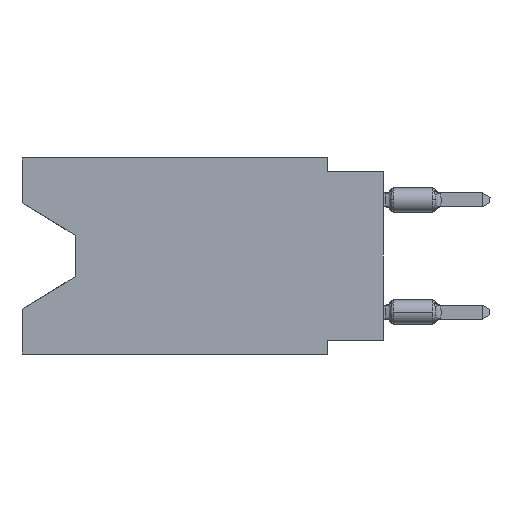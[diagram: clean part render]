
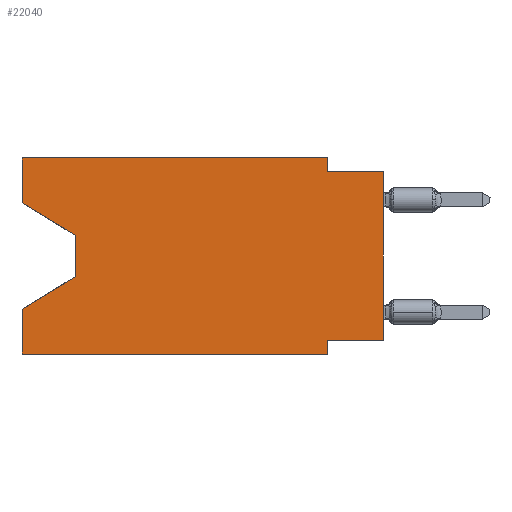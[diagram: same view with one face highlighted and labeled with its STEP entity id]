
A CAD part, left-side view. The second image highlights one B-rep face of the part: STEP entity #22040.
In plain terms, the highlighted planar face has unit normal (-1, 0, 0).
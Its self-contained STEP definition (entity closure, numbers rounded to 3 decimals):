
#743 = LINE ( 'NONE', #22579, #3223 ) ;
#1046 = LINE ( 'NONE', #13971, #13525 ) ;
#1055 = DIRECTION ( 'NONE',  ( 0., 0., 1. ) ) ;
#1995 = CARTESIAN_POINT ( 'NONE',  ( 0., 13.97, -5.385 ) ) ;
#2092 = CARTESIAN_POINT ( 'NONE',  ( 0., 16.383, 0. ) ) ;
#3223 = VECTOR ( 'NONE', #13660, 1000. ) ;
#3975 = LINE ( 'NONE', #13442, #32013 ) ;
#5871 = VERTEX_POINT ( 'NONE', #17220 ) ;
#7125 = ORIENTED_EDGE ( 'NONE', *, *, #10745, .T. ) ;
#7654 = VERTEX_POINT ( 'NONE', #24967 ) ;
#7940 = LINE ( 'NONE', #12248, #30791 ) ;
#9077 = LINE ( 'NONE', #12533, #16347 ) ;
#10044 = LINE ( 'NONE', #1995, #44112 ) ;
#10261 = ORIENTED_EDGE ( 'NONE', *, *, #47076, .T. ) ;
#10383 = CARTESIAN_POINT ( 'NONE',  ( 0., 16.383, -2.038 ) ) ;
#10745 = EDGE_CURVE ( 'NONE', #7654, #51484, #31964, .T. ) ;
#10991 = CARTESIAN_POINT ( 'NONE',  ( 0., 13.97, -3.505 ) ) ;
#11310 = CARTESIAN_POINT ( 'NONE',  ( 0., 2.54, 0. ) ) ;
#11563 = FACE_OUTER_BOUND ( 'NONE', #49711, .T. ) ;
#11608 = EDGE_CURVE ( 'NONE', #16523, #5871, #26941, .T. ) ;
#11979 = EDGE_CURVE ( 'NONE', #12028, #37269, #38691, .T. ) ;
#12028 = VERTEX_POINT ( 'NONE', #27717 ) ;
#12189 = CARTESIAN_POINT ( 'NONE',  ( 0., 2.54, -8.89 ) ) ;
#12248 = CARTESIAN_POINT ( 'NONE',  ( 0., 13.97, -3.505 ) ) ;
#12375 = EDGE_CURVE ( 'NONE', #30018, #5871, #10044, .T. ) ;
#12533 = CARTESIAN_POINT ( 'NONE',  ( 0., 16.383, 0. ) ) ;
#13442 = CARTESIAN_POINT ( 'NONE',  ( 0., 16.383, -8.89 ) ) ;
#13525 = VECTOR ( 'NONE', #22609, 1000. ) ;
#13660 = DIRECTION ( 'NONE',  ( 0., 0., 1. ) ) ;
#13665 = VECTOR ( 'NONE', #18730, 1000. ) ;
#13971 = CARTESIAN_POINT ( 'NONE',  ( 0., 0., -0.635 ) ) ;
#14748 = VERTEX_POINT ( 'NONE', #36480 ) ;
#15132 = EDGE_CURVE ( 'NONE', #36740, #51704, #41523, .T. ) ;
#15177 = EDGE_CURVE ( 'NONE', #12028, #49351, #51824, .T. ) ;
#15299 = DIRECTION ( 'NONE',  ( 1., 0., 0. ) ) ;
#16347 = VECTOR ( 'NONE', #16834, 1000. ) ;
#16513 = VECTOR ( 'NONE', #43290, 1000. ) ;
#16523 = VERTEX_POINT ( 'NONE', #43862 ) ;
#16834 = DIRECTION ( 'NONE',  ( 0., -1., 0. ) ) ;
#17220 = CARTESIAN_POINT ( 'NONE',  ( 0., 16.383, -6.852 ) ) ;
#18730 = DIRECTION ( 'NONE',  ( 0., -0.855, -0.519 ) ) ;
#19889 = ORIENTED_EDGE ( 'NONE', *, *, #15177, .T. ) ;
#20118 = VERTEX_POINT ( 'NONE', #34436 ) ;
#20897 = DIRECTION ( 'NONE',  ( 0., 0., -1. ) ) ;
#21114 = VECTOR ( 'NONE', #1055, 1000. ) ;
#22040 = ADVANCED_FACE ( 'NONE', ( #11563 ), #45507, .F. ) ;
#22579 = CARTESIAN_POINT ( 'NONE',  ( 0., 16.383, 0. ) ) ;
#22609 = DIRECTION ( 'NONE',  ( 0., -1., 0. ) ) ;
#24967 = CARTESIAN_POINT ( 'NONE',  ( 0., 16.383, -2.038 ) ) ;
#25403 = EDGE_CURVE ( 'NONE', #14748, #36740, #9077, .T. ) ;
#25697 = LINE ( 'NONE', #12189, #38447 ) ;
#26826 = VECTOR ( 'NONE', #52378, 1000. ) ;
#26941 = LINE ( 'NONE', #49068, #21114 ) ;
#27717 = CARTESIAN_POINT ( 'NONE',  ( 0., 0., -8.255 ) ) ;
#29427 = DIRECTION ( 'NONE',  ( 0., 0., -1. ) ) ;
#30018 = VERTEX_POINT ( 'NONE', #49094 ) ;
#30714 = EDGE_CURVE ( 'NONE', #37269, #20118, #25697, .T. ) ;
#30791 = VECTOR ( 'NONE', #20897, 1000. ) ;
#31431 = VECTOR ( 'NONE', #29427, 1000. ) ;
#31696 = ORIENTED_EDGE ( 'NONE', *, *, #25403, .F. ) ;
#31826 = AXIS2_PLACEMENT_3D ( 'NONE', #2092, #15299, #37749 ) ;
#31964 = LINE ( 'NONE', #10383, #13665 ) ;
#32013 = VECTOR ( 'NONE', #48527, 1000. ) ;
#34436 = CARTESIAN_POINT ( 'NONE',  ( 0., 2.54, -8.89 ) ) ;
#36480 = CARTESIAN_POINT ( 'NONE',  ( 0., 16.383, 0. ) ) ;
#36733 = ORIENTED_EDGE ( 'NONE', *, *, #11979, .F. ) ;
#36740 = VERTEX_POINT ( 'NONE', #53303 ) ;
#37269 = VERTEX_POINT ( 'NONE', #46584 ) ;
#37749 = DIRECTION ( 'NONE',  ( 0., 0., -1. ) ) ;
#38447 = VECTOR ( 'NONE', #42710, 1000. ) ;
#38691 = LINE ( 'NONE', #56780, #16513 ) ;
#38967 = EDGE_CURVE ( 'NONE', #7654, #14748, #743, .T. ) ;
#39242 = ORIENTED_EDGE ( 'NONE', *, *, #12375, .T. ) ;
#41523 = LINE ( 'NONE', #11310, #31431 ) ;
#42710 = DIRECTION ( 'NONE',  ( 0., 0., -1. ) ) ;
#42788 = ORIENTED_EDGE ( 'NONE', *, *, #38967, .F. ) ;
#43290 = DIRECTION ( 'NONE',  ( 0., 1., 0. ) ) ;
#43790 = ORIENTED_EDGE ( 'NONE', *, *, #30714, .F. ) ;
#43862 = CARTESIAN_POINT ( 'NONE',  ( 0., 16.383, -8.89 ) ) ;
#44112 = VECTOR ( 'NONE', #45124, 1000. ) ;
#44119 = EDGE_CURVE ( 'NONE', #16523, #20118, #3975, .T. ) ;
#44997 = ORIENTED_EDGE ( 'NONE', *, *, #44119, .T. ) ;
#45124 = DIRECTION ( 'NONE',  ( 0., 0.855, -0.519 ) ) ;
#45507 = PLANE ( 'NONE',  #31826 ) ;
#45558 = ORIENTED_EDGE ( 'NONE', *, *, #15132, .F. ) ;
#46584 = CARTESIAN_POINT ( 'NONE',  ( 0., 2.54, -8.255 ) ) ;
#47076 = EDGE_CURVE ( 'NONE', #51484, #30018, #7940, .T. ) ;
#47936 = ORIENTED_EDGE ( 'NONE', *, *, #11608, .F. ) ;
#48527 = DIRECTION ( 'NONE',  ( 0., -1., 0. ) ) ;
#49068 = CARTESIAN_POINT ( 'NONE',  ( 0., 16.383, 0. ) ) ;
#49094 = CARTESIAN_POINT ( 'NONE',  ( 0., 13.97, -5.385 ) ) ;
#49351 = VERTEX_POINT ( 'NONE', #53108 ) ;
#49711 = EDGE_LOOP ( 'NONE', ( #7125, #10261, #39242, #47936, #44997, #43790, #36733, #19889, #51087, #45558, #31696, #42788 ) ) ;
#51087 = ORIENTED_EDGE ( 'NONE', *, *, #55985, .F. ) ;
#51484 = VERTEX_POINT ( 'NONE', #10991 ) ;
#51704 = VERTEX_POINT ( 'NONE', #56368 ) ;
#51824 = LINE ( 'NONE', #52951, #26826 ) ;
#52378 = DIRECTION ( 'NONE',  ( 0., 0., 1. ) ) ;
#52951 = CARTESIAN_POINT ( 'NONE',  ( 0., 0., 0. ) ) ;
#53108 = CARTESIAN_POINT ( 'NONE',  ( 0., 0., -0.635 ) ) ;
#53303 = CARTESIAN_POINT ( 'NONE',  ( 0., 2.54, 0. ) ) ;
#55985 = EDGE_CURVE ( 'NONE', #51704, #49351, #1046, .T. ) ;
#56368 = CARTESIAN_POINT ( 'NONE',  ( 0., 2.54, -0.635 ) ) ;
#56780 = CARTESIAN_POINT ( 'NONE',  ( 0., 0., -8.255 ) ) ;
